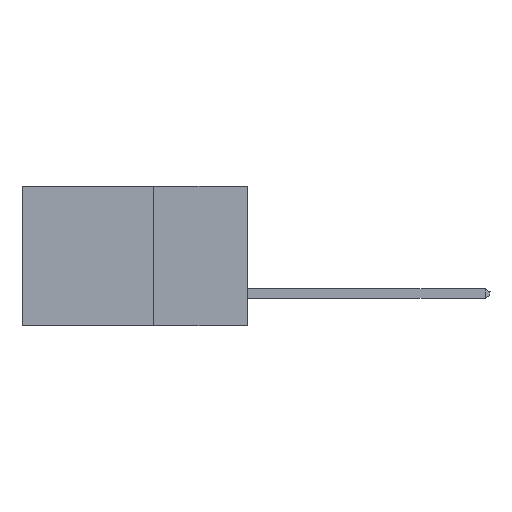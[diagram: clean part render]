
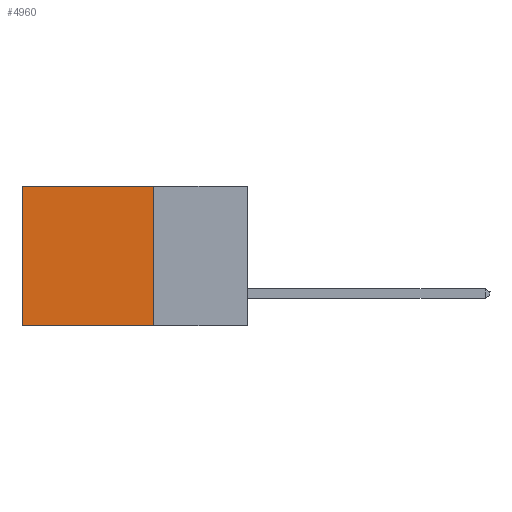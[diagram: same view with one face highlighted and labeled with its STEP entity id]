
A CAD part, left-side view. The second image highlights one B-rep face of the part: STEP entity #4960.
In plain terms, the highlighted planar face has unit normal (-1, 0, 0).
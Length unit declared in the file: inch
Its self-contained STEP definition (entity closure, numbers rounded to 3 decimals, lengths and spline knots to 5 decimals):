
#1294 = EDGE_CURVE ( 'NONE', #9622, #6560, #4017, .T. ) ;
#2941 = CARTESIAN_POINT ( 'NONE',  ( 0.2615, 0.25, -0.37 ) ) ;
#3098 = EDGE_CURVE ( 'NONE', #7230, #6560, #4569, .T. ) ;
#3214 = CARTESIAN_POINT ( 'NONE',  ( 0.2615, 0.6, -0.37 ) ) ;
#3223 = DIRECTION ( 'NONE',  ( 0., 0., -1. ) ) ;
#4017 = LINE ( 'NONE', #16853, #9159 ) ;
#4293 = CARTESIAN_POINT ( 'NONE',  ( 0.2615, 0.25, -0.37 ) ) ;
#4569 = LINE ( 'NONE', #16240, #15419 ) ;
#4925 = VECTOR ( 'NONE', #14431, 39.37008 ) ;
#4960 = ADVANCED_FACE ( 'NONE', ( #18252 ), #5110, .F. ) ;
#5110 = PLANE ( 'NONE',  #12710 ) ;
#5199 = DIRECTION ( 'NONE',  ( 0., 0., -1. ) ) ;
#6165 = ORIENTED_EDGE ( 'NONE', *, *, #17549, .F. ) ;
#6560 = VERTEX_POINT ( 'NONE', #3214 ) ;
#6637 = ORIENTED_EDGE ( 'NONE', *, *, #3098, .T. ) ;
#7230 = VERTEX_POINT ( 'NONE', #18522 ) ;
#8065 = DIRECTION ( 'NONE',  ( 1., 0., 0. ) ) ;
#9159 = VECTOR ( 'NONE', #9862, 39.37008 ) ;
#9622 = VERTEX_POINT ( 'NONE', #2941 ) ;
#9862 = DIRECTION ( 'NONE',  ( 0., 1., 0. ) ) ;
#10960 = CARTESIAN_POINT ( 'NONE',  ( 0.2615, 0.25, -0.37 ) ) ;
#12710 = AXIS2_PLACEMENT_3D ( 'NONE', #10960, #8065, #5199 ) ;
#14061 = DIRECTION ( 'NONE',  ( 0., 1., 0. ) ) ;
#14431 = DIRECTION ( 'NONE',  ( 0., 0., -1. ) ) ;
#14611 = VERTEX_POINT ( 'NONE', #18956 ) ;
#15034 = ORIENTED_EDGE ( 'NONE', *, *, #18370, .T. ) ;
#15419 = VECTOR ( 'NONE', #3223, 39.37008 ) ;
#16240 = CARTESIAN_POINT ( 'NONE',  ( 0.2615, 0.6, -0.37 ) ) ;
#16258 = VECTOR ( 'NONE', #14061, 39.37008 ) ;
#16416 = EDGE_LOOP ( 'NONE', ( #6637, #18755, #6165, #15034 ) ) ;
#16853 = CARTESIAN_POINT ( 'NONE',  ( 0.2615, 0.25, -0.37 ) ) ;
#17128 = LINE ( 'NONE', #18876, #16258 ) ;
#17549 = EDGE_CURVE ( 'NONE', #14611, #9622, #18774, .T. ) ;
#18252 = FACE_OUTER_BOUND ( 'NONE', #16416, .T. ) ;
#18370 = EDGE_CURVE ( 'NONE', #14611, #7230, #17128, .T. ) ;
#18522 = CARTESIAN_POINT ( 'NONE',  ( 0.2615, 0.6, 0. ) ) ;
#18755 = ORIENTED_EDGE ( 'NONE', *, *, #1294, .F. ) ;
#18774 = LINE ( 'NONE', #4293, #4925 ) ;
#18876 = CARTESIAN_POINT ( 'NONE',  ( 0.2615, 0.25, 0. ) ) ;
#18956 = CARTESIAN_POINT ( 'NONE',  ( 0.2615, 0.25, 0. ) ) ;
